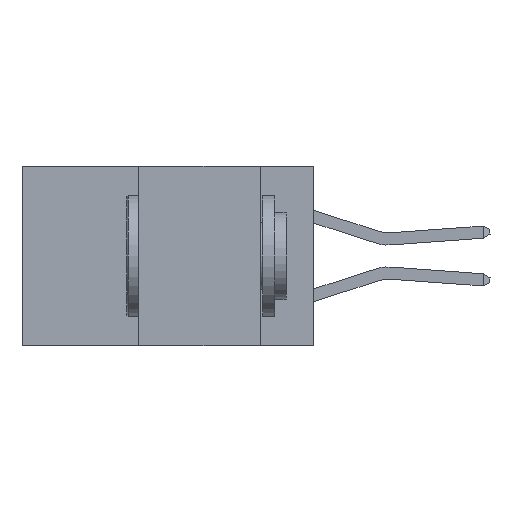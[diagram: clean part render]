
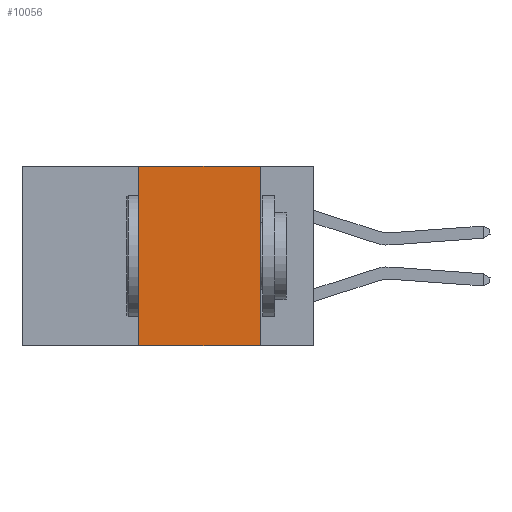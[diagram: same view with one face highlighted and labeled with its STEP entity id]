
A CAD part, left-side view. The second image highlights one B-rep face of the part: STEP entity #10056.
In plain terms, the highlighted planar face has unit normal (-1, 0, 0).
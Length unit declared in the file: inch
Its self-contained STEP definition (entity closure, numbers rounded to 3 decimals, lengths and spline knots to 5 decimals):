
#1264 = CARTESIAN_POINT ( 'NONE',  ( 0., 0.6, 0. ) ) ;
#3866 = DIRECTION ( 'NONE',  ( 1., 0., 0. ) ) ;
#6922 = DIRECTION ( 'NONE',  ( 0., 0., -1. ) ) ;
#7017 = CARTESIAN_POINT ( 'NONE',  ( 0., 0.11, 0. ) ) ;
#7228 = ORIENTED_EDGE ( 'NONE', *, *, #29701, .F. ) ;
#8365 = FACE_OUTER_BOUND ( 'NONE', #34741, .T. ) ;
#10056 = ADVANCED_FACE ( 'NONE', ( #8365 ), #35136, .F. ) ;
#11094 = DIRECTION ( 'NONE',  ( 0., -1., 0. ) ) ;
#12777 = CARTESIAN_POINT ( 'NONE',  ( 0., 0.11, 0. ) ) ;
#13205 = CARTESIAN_POINT ( 'NONE',  ( 0., 0.6, -0.37 ) ) ;
#13316 = VECTOR ( 'NONE', #6922, 39.37008 ) ;
#15761 = VERTEX_POINT ( 'NONE', #17479 ) ;
#16387 = CARTESIAN_POINT ( 'NONE',  ( 0., 0.11, -0.37 ) ) ;
#17166 = VECTOR ( 'NONE', #11094, 39.37008 ) ;
#17479 = CARTESIAN_POINT ( 'NONE',  ( 0., 0.36, -0.37 ) ) ;
#19710 = LINE ( 'NONE', #12777, #13316 ) ;
#20769 = VERTEX_POINT ( 'NONE', #38066 ) ;
#21110 = AXIS2_PLACEMENT_3D ( 'NONE', #38247, #3866, #32228 ) ;
#22760 = CARTESIAN_POINT ( 'NONE',  ( 0., 0.36, 0. ) ) ;
#25241 = ORIENTED_EDGE ( 'NONE', *, *, #36231, .T. ) ;
#25524 = DIRECTION ( 'NONE',  ( 0., -1., 0. ) ) ;
#27920 = LINE ( 'NONE', #13205, #30365 ) ;
#28468 = EDGE_CURVE ( 'NONE', #29372, #36382, #19710, .T. ) ;
#29372 = VERTEX_POINT ( 'NONE', #7017 ) ;
#29701 = EDGE_CURVE ( 'NONE', #20769, #29372, #31028, .T. ) ;
#30365 = VECTOR ( 'NONE', #25524, 39.37008 ) ;
#31028 = LINE ( 'NONE', #1264, #17166 ) ;
#32228 = DIRECTION ( 'NONE',  ( 0., 0., -1. ) ) ;
#34741 = EDGE_LOOP ( 'NONE', ( #40947, #7228, #36443, #25241 ) ) ;
#34885 = LINE ( 'NONE', #22760, #36381 ) ;
#35136 = PLANE ( 'NONE',  #21110 ) ;
#36231 = EDGE_CURVE ( 'NONE', #15761, #36382, #27920, .T. ) ;
#36381 = VECTOR ( 'NONE', #38200, 39.37008 ) ;
#36382 = VERTEX_POINT ( 'NONE', #16387 ) ;
#36443 = ORIENTED_EDGE ( 'NONE', *, *, #40506, .F. ) ;
#38066 = CARTESIAN_POINT ( 'NONE',  ( 0., 0.36, 0. ) ) ;
#38200 = DIRECTION ( 'NONE',  ( 0., 0., 1. ) ) ;
#38247 = CARTESIAN_POINT ( 'NONE',  ( 0., 0.6, 0. ) ) ;
#40506 = EDGE_CURVE ( 'NONE', #15761, #20769, #34885, .T. ) ;
#40947 = ORIENTED_EDGE ( 'NONE', *, *, #28468, .F. ) ;
